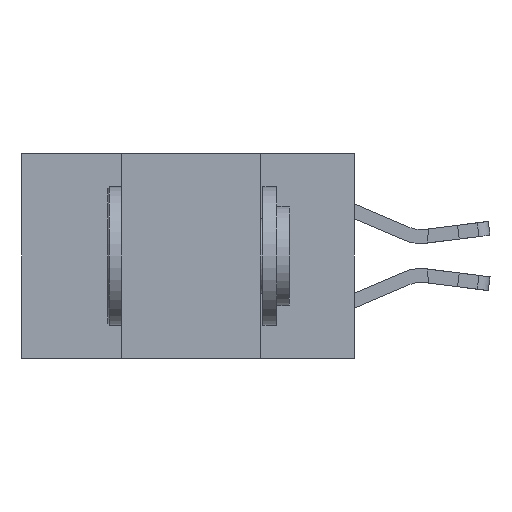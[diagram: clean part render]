
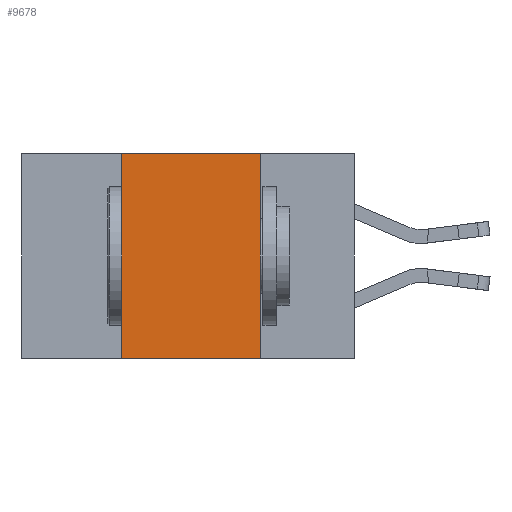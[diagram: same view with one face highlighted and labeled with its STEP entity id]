
A CAD part, left-side view. The second image highlights one B-rep face of the part: STEP entity #9678.
In plain terms, the highlighted planar face has unit normal (-1, 0, 0).
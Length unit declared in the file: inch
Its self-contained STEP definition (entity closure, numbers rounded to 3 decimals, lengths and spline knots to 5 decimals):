
#131 = CARTESIAN_POINT ( 'NONE',  ( 0., 0.17, 0. ) ) ;
#238 = ORIENTED_EDGE ( 'NONE', *, *, #12026, .F. ) ;
#516 = LINE ( 'NONE', #13880, #19031 ) ;
#1454 = EDGE_CURVE ( 'NONE', #7450, #12863, #516, .T. ) ;
#1840 = VECTOR ( 'NONE', #9943, 39.37008 ) ;
#2225 = AXIS2_PLACEMENT_3D ( 'NONE', #13398, #4027, #17489 ) ;
#2227 = PLANE ( 'NONE',  #2225 ) ;
#2881 = ORIENTED_EDGE ( 'NONE', *, *, #12388, .T. ) ;
#4027 = DIRECTION ( 'NONE',  ( 1., 0., 0. ) ) ;
#4501 = VECTOR ( 'NONE', #22744, 39.37008 ) ;
#6323 = EDGE_CURVE ( 'NONE', #6923, #8435, #8075, .T. ) ;
#6904 = LINE ( 'NONE', #15649, #1840 ) ;
#6923 = VERTEX_POINT ( 'NONE', #23012 ) ;
#7450 = VERTEX_POINT ( 'NONE', #131 ) ;
#8075 = LINE ( 'NONE', #18726, #4501 ) ;
#8232 = CARTESIAN_POINT ( 'NONE',  ( 0., 0.6, 0. ) ) ;
#8435 = VERTEX_POINT ( 'NONE', #10693 ) ;
#9678 = ADVANCED_FACE ( 'NONE', ( #24572 ), #2227, .F. ) ;
#9943 = DIRECTION ( 'NONE',  ( 0., -1., 0. ) ) ;
#10693 = CARTESIAN_POINT ( 'NONE',  ( 0., 0.42, 0. ) ) ;
#12026 = EDGE_CURVE ( 'NONE', #8435, #7450, #12595, .T. ) ;
#12054 = ORIENTED_EDGE ( 'NONE', *, *, #1454, .F. ) ;
#12388 = EDGE_CURVE ( 'NONE', #6923, #12863, #6904, .T. ) ;
#12595 = LINE ( 'NONE', #8232, #15859 ) ;
#12863 = VERTEX_POINT ( 'NONE', #14971 ) ;
#13398 = CARTESIAN_POINT ( 'NONE',  ( 0., 0.6, 0. ) ) ;
#13880 = CARTESIAN_POINT ( 'NONE',  ( 0., 0.17, 0. ) ) ;
#14971 = CARTESIAN_POINT ( 'NONE',  ( 0., 0.17, -0.37 ) ) ;
#15649 = CARTESIAN_POINT ( 'NONE',  ( 0., 0.6, -0.37 ) ) ;
#15859 = VECTOR ( 'NONE', #24027, 39.37008 ) ;
#17489 = DIRECTION ( 'NONE',  ( 0., 0., -1. ) ) ;
#18726 = CARTESIAN_POINT ( 'NONE',  ( 0., 0.42, 0. ) ) ;
#19031 = VECTOR ( 'NONE', #19774, 39.37008 ) ;
#19774 = DIRECTION ( 'NONE',  ( 0., 0., -1. ) ) ;
#22382 = EDGE_LOOP ( 'NONE', ( #12054, #238, #24522, #2881 ) ) ;
#22744 = DIRECTION ( 'NONE',  ( 0., 0., 1. ) ) ;
#23012 = CARTESIAN_POINT ( 'NONE',  ( 0., 0.42, -0.37 ) ) ;
#24027 = DIRECTION ( 'NONE',  ( 0., -1., 0. ) ) ;
#24522 = ORIENTED_EDGE ( 'NONE', *, *, #6323, .F. ) ;
#24572 = FACE_OUTER_BOUND ( 'NONE', #22382, .T. ) ;
